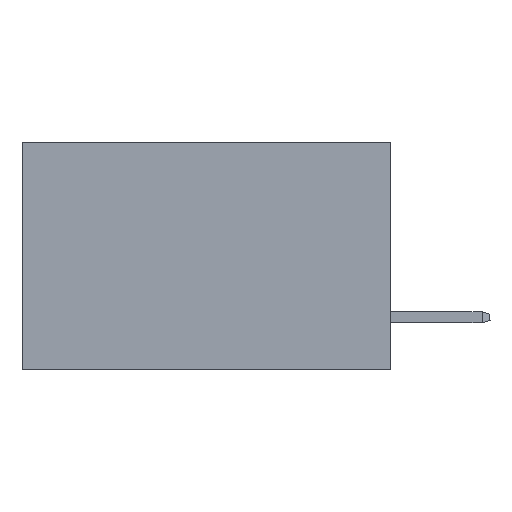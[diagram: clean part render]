
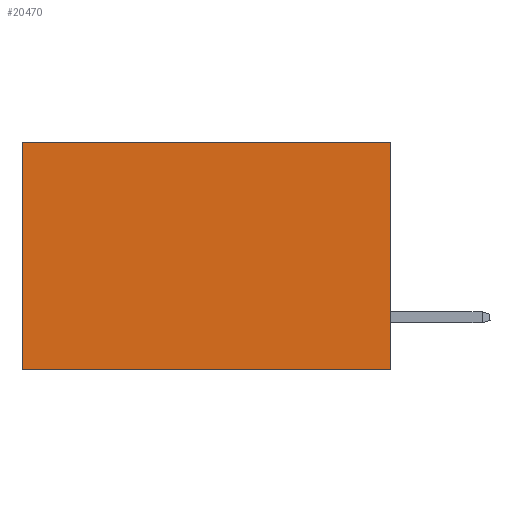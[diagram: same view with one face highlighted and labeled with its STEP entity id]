
A CAD part, left-side view. The second image highlights one B-rep face of the part: STEP entity #20470.
In plain terms, the highlighted planar face has unit normal (-1, 0, 0).
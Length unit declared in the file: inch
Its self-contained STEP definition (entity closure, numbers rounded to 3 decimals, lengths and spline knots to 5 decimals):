
#487 = DIRECTION ( 'NONE',  ( 0., 1., 0. ) ) ;
#663 = CARTESIAN_POINT ( 'NONE',  ( 0.2875, 0., 0. ) ) ;
#792 = VERTEX_POINT ( 'NONE', #18622 ) ;
#2258 = ORIENTED_EDGE ( 'NONE', *, *, #11391, .F. ) ;
#2304 = DIRECTION ( 'NONE',  ( 0., 0., -1. ) ) ;
#2400 = LINE ( 'NONE', #5515, #14598 ) ;
#2448 = ORIENTED_EDGE ( 'NONE', *, *, #11142, .F. ) ;
#2786 = VECTOR ( 'NONE', #12790, 39.37008 ) ;
#3200 = VECTOR ( 'NONE', #8362, 39.37008 ) ;
#4661 = VERTEX_POINT ( 'NONE', #15085 ) ;
#5051 = VERTEX_POINT ( 'NONE', #5448 ) ;
#5448 = CARTESIAN_POINT ( 'NONE',  ( 0.2875, 0., -0.37 ) ) ;
#5515 = CARTESIAN_POINT ( 'NONE',  ( 0.2875, 0., 0. ) ) ;
#5600 = VERTEX_POINT ( 'NONE', #8704 ) ;
#6922 = CARTESIAN_POINT ( 'NONE',  ( 0.2875, 0., 0. ) ) ;
#8285 = LINE ( 'NONE', #6922, #12408 ) ;
#8362 = DIRECTION ( 'NONE',  ( 0., 0., -1. ) ) ;
#8509 = CARTESIAN_POINT ( 'NONE',  ( 0.2875, 0.6, 0. ) ) ;
#8704 = CARTESIAN_POINT ( 'NONE',  ( 0.2875, 0.6, -0.37 ) ) ;
#8994 = DIRECTION ( 'NONE',  ( 1., 0., 0. ) ) ;
#9140 = FACE_OUTER_BOUND ( 'NONE', #13056, .T. ) ;
#9424 = LINE ( 'NONE', #8509, #3200 ) ;
#11142 = EDGE_CURVE ( 'NONE', #792, #5051, #8285, .T. ) ;
#11391 = EDGE_CURVE ( 'NONE', #5051, #5600, #16802, .T. ) ;
#12408 = VECTOR ( 'NONE', #18414, 39.37008 ) ;
#12790 = DIRECTION ( 'NONE',  ( 0., 1., 0. ) ) ;
#13056 = EDGE_LOOP ( 'NONE', ( #17816, #2258, #2448, #19681 ) ) ;
#13774 = EDGE_CURVE ( 'NONE', #792, #4661, #2400, .T. ) ;
#14231 = EDGE_CURVE ( 'NONE', #4661, #5600, #9424, .T. ) ;
#14598 = VECTOR ( 'NONE', #487, 39.37008 ) ;
#15085 = CARTESIAN_POINT ( 'NONE',  ( 0.2875, 0.6, 0. ) ) ;
#15642 = PLANE ( 'NONE',  #18937 ) ;
#16802 = LINE ( 'NONE', #17814, #2786 ) ;
#17814 = CARTESIAN_POINT ( 'NONE',  ( 0.2875, 0., -0.37 ) ) ;
#17816 = ORIENTED_EDGE ( 'NONE', *, *, #14231, .T. ) ;
#18414 = DIRECTION ( 'NONE',  ( 0., 0., -1. ) ) ;
#18622 = CARTESIAN_POINT ( 'NONE',  ( 0.2875, 0., 0. ) ) ;
#18937 = AXIS2_PLACEMENT_3D ( 'NONE', #663, #8994, #2304 ) ;
#19681 = ORIENTED_EDGE ( 'NONE', *, *, #13774, .T. ) ;
#20470 = ADVANCED_FACE ( 'NONE', ( #9140 ), #15642, .F. ) ;
